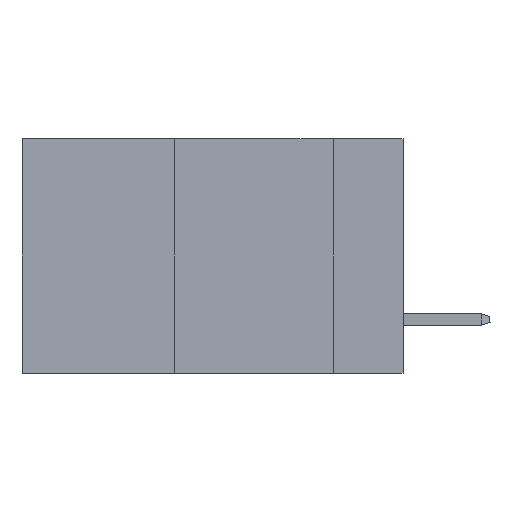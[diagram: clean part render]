
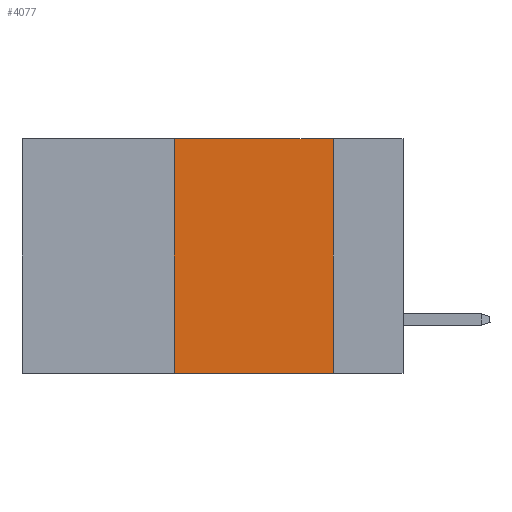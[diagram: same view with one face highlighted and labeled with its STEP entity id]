
A CAD part, left-side view. The second image highlights one B-rep face of the part: STEP entity #4077.
In plain terms, the highlighted planar face has unit normal (-1, 0, 0).
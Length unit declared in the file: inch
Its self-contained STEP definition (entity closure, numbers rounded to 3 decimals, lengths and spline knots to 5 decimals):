
#282 = VERTEX_POINT ( 'NONE', #4754 ) ;
#468 = CARTESIAN_POINT ( 'NONE',  ( 0., 0.11, 0. ) ) ;
#1414 = EDGE_CURVE ( 'NONE', #12131, #10991, #20174, .T. ) ;
#1659 = EDGE_LOOP ( 'NONE', ( #15632, #13468, #15282, #3386 ) ) ;
#2094 = VECTOR ( 'NONE', #18009, 39.37008 ) ;
#2454 = VERTEX_POINT ( 'NONE', #468 ) ;
#2508 = PLANE ( 'NONE',  #15424 ) ;
#2621 = EDGE_CURVE ( 'NONE', #282, #2454, #4642, .T. ) ;
#2885 = DIRECTION ( 'NONE',  ( 0., 0., -1. ) ) ;
#3041 = VECTOR ( 'NONE', #2885, 39.37008 ) ;
#3359 = DIRECTION ( 'NONE',  ( 0., -1., 0. ) ) ;
#3386 = ORIENTED_EDGE ( 'NONE', *, *, #1414, .T. ) ;
#3437 = VECTOR ( 'NONE', #14873, 39.37008 ) ;
#4077 = ADVANCED_FACE ( 'NONE', ( #12457 ), #2508, .F. ) ;
#4642 = LINE ( 'NONE', #17907, #2094 ) ;
#4754 = CARTESIAN_POINT ( 'NONE',  ( 0., 0.36, 0. ) ) ;
#7182 = DIRECTION ( 'NONE',  ( 1., 0., 0. ) ) ;
#10035 = LINE ( 'NONE', #13559, #3437 ) ;
#10930 = CARTESIAN_POINT ( 'NONE',  ( 0., 0.6, 0. ) ) ;
#10991 = VERTEX_POINT ( 'NONE', #12838 ) ;
#12131 = VERTEX_POINT ( 'NONE', #12524 ) ;
#12457 = FACE_OUTER_BOUND ( 'NONE', #1659, .T. ) ;
#12524 = CARTESIAN_POINT ( 'NONE',  ( 0., 0.36, -0.37 ) ) ;
#12838 = CARTESIAN_POINT ( 'NONE',  ( 0., 0.11, -0.37 ) ) ;
#13159 = CARTESIAN_POINT ( 'NONE',  ( 0., 0.11, 0. ) ) ;
#13468 = ORIENTED_EDGE ( 'NONE', *, *, #2621, .F. ) ;
#13559 = CARTESIAN_POINT ( 'NONE',  ( 0., 0.36, 0. ) ) ;
#13897 = DIRECTION ( 'NONE',  ( 0., 0., -1. ) ) ;
#14873 = DIRECTION ( 'NONE',  ( 0., 0., 1. ) ) ;
#15282 = ORIENTED_EDGE ( 'NONE', *, *, #20108, .F. ) ;
#15424 = AXIS2_PLACEMENT_3D ( 'NONE', #10930, #7182, #13897 ) ;
#15632 = ORIENTED_EDGE ( 'NONE', *, *, #17396, .F. ) ;
#16481 = LINE ( 'NONE', #13159, #3041 ) ;
#17396 = EDGE_CURVE ( 'NONE', #2454, #10991, #16481, .T. ) ;
#17907 = CARTESIAN_POINT ( 'NONE',  ( 0., 0.6, 0. ) ) ;
#18009 = DIRECTION ( 'NONE',  ( 0., -1., 0. ) ) ;
#18612 = CARTESIAN_POINT ( 'NONE',  ( 0., 0.6, -0.37 ) ) ;
#20108 = EDGE_CURVE ( 'NONE', #12131, #282, #10035, .T. ) ;
#20144 = VECTOR ( 'NONE', #3359, 39.37008 ) ;
#20174 = LINE ( 'NONE', #18612, #20144 ) ;
